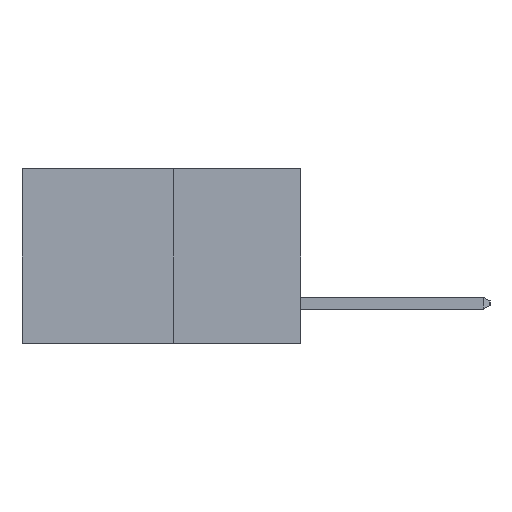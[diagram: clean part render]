
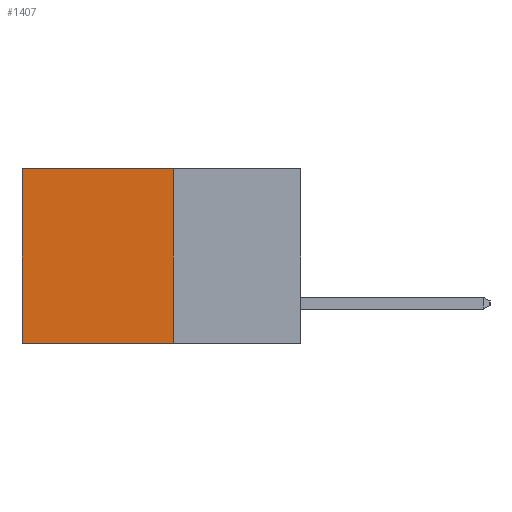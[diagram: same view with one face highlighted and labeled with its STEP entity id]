
A CAD part, left-side view. The second image highlights one B-rep face of the part: STEP entity #1407.
In plain terms, the highlighted planar face has unit normal (-1, 0, 0).
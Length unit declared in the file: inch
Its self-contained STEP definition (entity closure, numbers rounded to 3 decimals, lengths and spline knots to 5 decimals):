
#199 = PLANE ( 'NONE',  #5866 ) ;
#226 = EDGE_CURVE ( 'NONE', #4090, #4696, #10855, .T. ) ;
#267 = VERTEX_POINT ( 'NONE', #6487 ) ;
#288 = ORIENTED_EDGE ( 'NONE', *, *, #226, .F. ) ;
#963 = DIRECTION ( 'NONE',  ( 0., 0., -1. ) ) ;
#1103 = CARTESIAN_POINT ( 'NONE',  ( 0.277, 0.27, -0.37 ) ) ;
#1407 = ADVANCED_FACE ( 'NONE', ( #7794 ), #199, .F. ) ;
#1592 = VECTOR ( 'NONE', #8479, 39.37008 ) ;
#2440 = CARTESIAN_POINT ( 'NONE',  ( 0.277, 0.27, -0.37 ) ) ;
#2641 = LINE ( 'NONE', #9448, #4495 ) ;
#2953 = CARTESIAN_POINT ( 'NONE',  ( 0.277, 0.27, 0. ) ) ;
#4090 = VERTEX_POINT ( 'NONE', #9483 ) ;
#4398 = DIRECTION ( 'NONE',  ( 0., 1., 0. ) ) ;
#4495 = VECTOR ( 'NONE', #8815, 39.37008 ) ;
#4598 = DIRECTION ( 'NONE',  ( 0., 0., -1. ) ) ;
#4696 = VERTEX_POINT ( 'NONE', #9759 ) ;
#5068 = VECTOR ( 'NONE', #4398, 39.37008 ) ;
#5866 = AXIS2_PLACEMENT_3D ( 'NONE', #2440, #6404, #4598 ) ;
#5883 = EDGE_CURVE ( 'NONE', #4090, #267, #7627, .T. ) ;
#6030 = CARTESIAN_POINT ( 'NONE',  ( 0.277, 0.59, -0.37 ) ) ;
#6289 = EDGE_CURVE ( 'NONE', #4696, #6319, #2641, .T. ) ;
#6319 = VERTEX_POINT ( 'NONE', #8386 ) ;
#6404 = DIRECTION ( 'NONE',  ( 1., 0., 0. ) ) ;
#6487 = CARTESIAN_POINT ( 'NONE',  ( 0.277, 0.59, 0. ) ) ;
#7627 = LINE ( 'NONE', #2953, #5068 ) ;
#7794 = FACE_OUTER_BOUND ( 'NONE', #8159, .T. ) ;
#8089 = EDGE_CURVE ( 'NONE', #267, #6319, #8307, .T. ) ;
#8159 = EDGE_LOOP ( 'NONE', ( #8708, #8312, #288, #9016 ) ) ;
#8307 = LINE ( 'NONE', #6030, #1592 ) ;
#8312 = ORIENTED_EDGE ( 'NONE', *, *, #6289, .F. ) ;
#8386 = CARTESIAN_POINT ( 'NONE',  ( 0.277, 0.59, -0.37 ) ) ;
#8479 = DIRECTION ( 'NONE',  ( 0., 0., -1. ) ) ;
#8708 = ORIENTED_EDGE ( 'NONE', *, *, #8089, .T. ) ;
#8815 = DIRECTION ( 'NONE',  ( 0., 1., 0. ) ) ;
#8976 = VECTOR ( 'NONE', #963, 39.37008 ) ;
#9016 = ORIENTED_EDGE ( 'NONE', *, *, #5883, .T. ) ;
#9448 = CARTESIAN_POINT ( 'NONE',  ( 0.277, 0.27, -0.37 ) ) ;
#9483 = CARTESIAN_POINT ( 'NONE',  ( 0.277, 0.27, 0. ) ) ;
#9759 = CARTESIAN_POINT ( 'NONE',  ( 0.277, 0.27, -0.37 ) ) ;
#10855 = LINE ( 'NONE', #1103, #8976 ) ;
